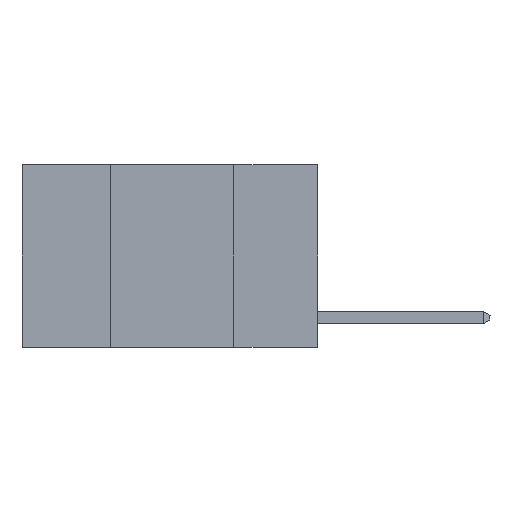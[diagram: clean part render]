
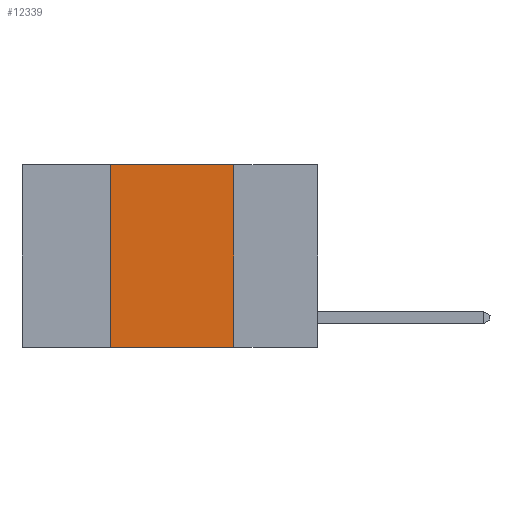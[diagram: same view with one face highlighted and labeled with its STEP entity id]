
A CAD part, left-side view. The second image highlights one B-rep face of the part: STEP entity #12339.
In plain terms, the highlighted planar face has unit normal (-1, 0, 0).
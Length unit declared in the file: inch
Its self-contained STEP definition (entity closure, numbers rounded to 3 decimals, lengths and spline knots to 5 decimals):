
#295 = LINE ( 'NONE', #11950, #3503 ) ;
#688 = CARTESIAN_POINT ( 'NONE',  ( 0., 0.6, -0.37 ) ) ;
#719 = ORIENTED_EDGE ( 'NONE', *, *, #3867, .T. ) ;
#846 = PLANE ( 'NONE',  #6909 ) ;
#1183 = CARTESIAN_POINT ( 'NONE',  ( 0., 0.42, -0.37 ) ) ;
#1370 = LINE ( 'NONE', #688, #6689 ) ;
#1554 = VERTEX_POINT ( 'NONE', #1183 ) ;
#1567 = DIRECTION ( 'NONE',  ( 0., -1., 0. ) ) ;
#1918 = LINE ( 'NONE', #7107, #11005 ) ;
#2385 = CARTESIAN_POINT ( 'NONE',  ( 0., 0.17, 0. ) ) ;
#2470 = DIRECTION ( 'NONE',  ( 0., 0., 1. ) ) ;
#2830 = ORIENTED_EDGE ( 'NONE', *, *, #4930, .F. ) ;
#3083 = VERTEX_POINT ( 'NONE', #3456 ) ;
#3456 = CARTESIAN_POINT ( 'NONE',  ( 0., 0.17, -0.37 ) ) ;
#3464 = CARTESIAN_POINT ( 'NONE',  ( 0., 0.6, 0. ) ) ;
#3503 = VECTOR ( 'NONE', #6148, 39.37008 ) ;
#3867 = EDGE_CURVE ( 'NONE', #1554, #3083, #1370, .T. ) ;
#4476 = VERTEX_POINT ( 'NONE', #2385 ) ;
#4930 = EDGE_CURVE ( 'NONE', #4476, #3083, #295, .T. ) ;
#6148 = DIRECTION ( 'NONE',  ( 0., 0., -1. ) ) ;
#6335 = EDGE_CURVE ( 'NONE', #1554, #7655, #1918, .T. ) ;
#6406 = DIRECTION ( 'NONE',  ( 0., -1., 0. ) ) ;
#6535 = EDGE_CURVE ( 'NONE', #7655, #4476, #8587, .T. ) ;
#6689 = VECTOR ( 'NONE', #1567, 39.37008 ) ;
#6702 = ORIENTED_EDGE ( 'NONE', *, *, #6535, .F. ) ;
#6909 = AXIS2_PLACEMENT_3D ( 'NONE', #8698, #10594, #10434 ) ;
#7107 = CARTESIAN_POINT ( 'NONE',  ( 0., 0.42, 0. ) ) ;
#7655 = VERTEX_POINT ( 'NONE', #11623 ) ;
#8587 = LINE ( 'NONE', #3464, #9650 ) ;
#8698 = CARTESIAN_POINT ( 'NONE',  ( 0., 0.6, 0. ) ) ;
#9134 = FACE_OUTER_BOUND ( 'NONE', #9425, .T. ) ;
#9425 = EDGE_LOOP ( 'NONE', ( #2830, #6702, #10776, #719 ) ) ;
#9650 = VECTOR ( 'NONE', #6406, 39.37008 ) ;
#10434 = DIRECTION ( 'NONE',  ( 0., 0., -1. ) ) ;
#10594 = DIRECTION ( 'NONE',  ( 1., 0., 0. ) ) ;
#10776 = ORIENTED_EDGE ( 'NONE', *, *, #6335, .F. ) ;
#11005 = VECTOR ( 'NONE', #2470, 39.37008 ) ;
#11623 = CARTESIAN_POINT ( 'NONE',  ( 0., 0.42, 0. ) ) ;
#11950 = CARTESIAN_POINT ( 'NONE',  ( 0., 0.17, 0. ) ) ;
#12339 = ADVANCED_FACE ( 'NONE', ( #9134 ), #846, .F. ) ;
